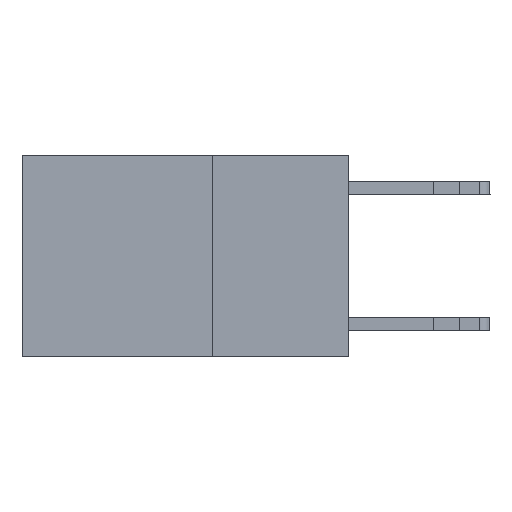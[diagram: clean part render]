
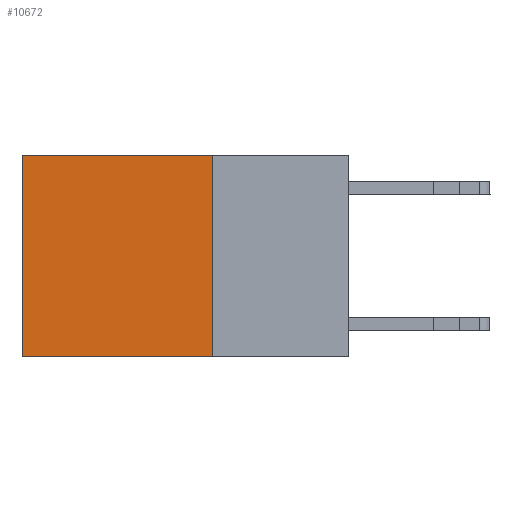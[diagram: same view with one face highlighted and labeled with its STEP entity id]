
A CAD part, left-side view. The second image highlights one B-rep face of the part: STEP entity #10672.
In plain terms, the highlighted planar face has unit normal (-1, 0, 0).
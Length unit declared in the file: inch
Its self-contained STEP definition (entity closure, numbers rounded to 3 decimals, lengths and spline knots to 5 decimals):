
#194 = VERTEX_POINT ( 'NONE', #13506 ) ;
#292 = CARTESIAN_POINT ( 'NONE',  ( 0.2625, 0.6, 0. ) ) ;
#1358 = DIRECTION ( 'NONE',  ( 1., 0., 0. ) ) ;
#1365 = VECTOR ( 'NONE', #9566, 39.37008 ) ;
#1445 = EDGE_CURVE ( 'NONE', #194, #8638, #15204, .T. ) ;
#1757 = LINE ( 'NONE', #9966, #1901 ) ;
#1862 = DIRECTION ( 'NONE',  ( 0., 0., -1. ) ) ;
#1901 = VECTOR ( 'NONE', #14052, 39.37008 ) ;
#2760 = LINE ( 'NONE', #292, #1365 ) ;
#2878 = VERTEX_POINT ( 'NONE', #7724 ) ;
#4013 = EDGE_CURVE ( 'NONE', #194, #8864, #5511, .T. ) ;
#5356 = CARTESIAN_POINT ( 'NONE',  ( 0.2625, 0.25, -0.37 ) ) ;
#5424 = CARTESIAN_POINT ( 'NONE',  ( 0.2625, 0.25, 0. ) ) ;
#5511 = LINE ( 'NONE', #10972, #11160 ) ;
#5810 = ORIENTED_EDGE ( 'NONE', *, *, #6535, .F. ) ;
#6535 = EDGE_CURVE ( 'NONE', #8638, #2878, #1757, .T. ) ;
#6767 = FACE_OUTER_BOUND ( 'NONE', #10850, .T. ) ;
#7376 = AXIS2_PLACEMENT_3D ( 'NONE', #5424, #1358, #10883 ) ;
#7413 = VECTOR ( 'NONE', #1862, 39.37008 ) ;
#7724 = CARTESIAN_POINT ( 'NONE',  ( 0.2625, 0.6, -0.37 ) ) ;
#8638 = VERTEX_POINT ( 'NONE', #5356 ) ;
#8864 = VERTEX_POINT ( 'NONE', #10696 ) ;
#9566 = DIRECTION ( 'NONE',  ( 0., 0., -1. ) ) ;
#9895 = CARTESIAN_POINT ( 'NONE',  ( 0.2625, 0.25, 0. ) ) ;
#9966 = CARTESIAN_POINT ( 'NONE',  ( 0.2625, 0.25, -0.37 ) ) ;
#10672 = ADVANCED_FACE ( 'NONE', ( #6767 ), #16285, .F. ) ;
#10696 = CARTESIAN_POINT ( 'NONE',  ( 0.2625, 0.6, 0. ) ) ;
#10850 = EDGE_LOOP ( 'NONE', ( #13712, #5810, #12892, #15317 ) ) ;
#10883 = DIRECTION ( 'NONE',  ( 0., 0., -1. ) ) ;
#10972 = CARTESIAN_POINT ( 'NONE',  ( 0.2625, 0.25, 0. ) ) ;
#11160 = VECTOR ( 'NONE', #16184, 39.37008 ) ;
#12645 = EDGE_CURVE ( 'NONE', #8864, #2878, #2760, .T. ) ;
#12892 = ORIENTED_EDGE ( 'NONE', *, *, #1445, .F. ) ;
#13506 = CARTESIAN_POINT ( 'NONE',  ( 0.2625, 0.25, 0. ) ) ;
#13712 = ORIENTED_EDGE ( 'NONE', *, *, #12645, .T. ) ;
#14052 = DIRECTION ( 'NONE',  ( 0., 1., 0. ) ) ;
#15204 = LINE ( 'NONE', #9895, #7413 ) ;
#15317 = ORIENTED_EDGE ( 'NONE', *, *, #4013, .T. ) ;
#16184 = DIRECTION ( 'NONE',  ( 0., 1., 0. ) ) ;
#16285 = PLANE ( 'NONE',  #7376 ) ;
